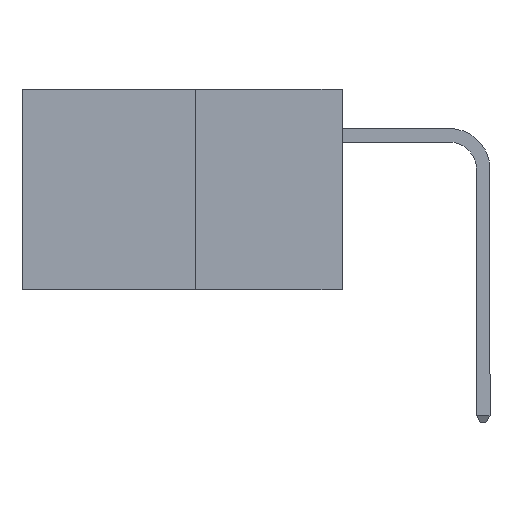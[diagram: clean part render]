
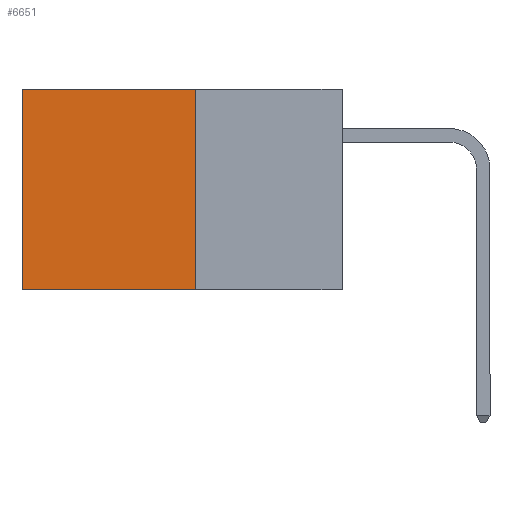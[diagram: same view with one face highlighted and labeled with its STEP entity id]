
A CAD part, left-side view. The second image highlights one B-rep face of the part: STEP entity #6651.
In plain terms, the highlighted planar face has unit normal (-1, 0, 0).
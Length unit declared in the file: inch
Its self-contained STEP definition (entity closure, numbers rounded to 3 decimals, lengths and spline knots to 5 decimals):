
#1680 = DIRECTION ( 'NONE',  ( 0., 0., -1. ) ) ;
#1918 = VERTEX_POINT ( 'NONE', #6724 ) ;
#2321 = VERTEX_POINT ( 'NONE', #21889 ) ;
#2814 = VERTEX_POINT ( 'NONE', #12919 ) ;
#4074 = DIRECTION ( 'NONE',  ( 0., 1., 0. ) ) ;
#5026 = EDGE_CURVE ( 'NONE', #2814, #1918, #20835, .T. ) ;
#5710 = ORIENTED_EDGE ( 'NONE', *, *, #10222, .F. ) ;
#6615 = LINE ( 'NONE', #10539, #15986 ) ;
#6651 = ADVANCED_FACE ( 'NONE', ( #14826 ), #9580, .F. ) ;
#6724 = CARTESIAN_POINT ( 'NONE',  ( 0.277, 0.59, 0. ) ) ;
#8294 = AXIS2_PLACEMENT_3D ( 'NONE', #15497, #8784, #8706 ) ;
#8706 = DIRECTION ( 'NONE',  ( 0., 0., -1. ) ) ;
#8784 = DIRECTION ( 'NONE',  ( 1., 0., 0. ) ) ;
#9580 = PLANE ( 'NONE',  #8294 ) ;
#9898 = CARTESIAN_POINT ( 'NONE',  ( 0.277, 0.27, 0. ) ) ;
#9905 = CARTESIAN_POINT ( 'NONE',  ( 0.277, 0.59, -0.37 ) ) ;
#10222 = EDGE_CURVE ( 'NONE', #2321, #20116, #14218, .T. ) ;
#10539 = CARTESIAN_POINT ( 'NONE',  ( 0.277, 0.27, -0.37 ) ) ;
#11614 = VECTOR ( 'NONE', #16657, 39.37008 ) ;
#11790 = EDGE_LOOP ( 'NONE', ( #13948, #5710, #15929, #20528 ) ) ;
#12919 = CARTESIAN_POINT ( 'NONE',  ( 0.277, 0.27, 0. ) ) ;
#13169 = CARTESIAN_POINT ( 'NONE',  ( 0.277, 0.59, -0.37 ) ) ;
#13433 = DIRECTION ( 'NONE',  ( 0., 0., -1. ) ) ;
#13948 = ORIENTED_EDGE ( 'NONE', *, *, #19528, .T. ) ;
#14218 = LINE ( 'NONE', #18161, #18277 ) ;
#14826 = FACE_OUTER_BOUND ( 'NONE', #11790, .T. ) ;
#15497 = CARTESIAN_POINT ( 'NONE',  ( 0.277, 0.27, -0.37 ) ) ;
#15929 = ORIENTED_EDGE ( 'NONE', *, *, #21591, .F. ) ;
#15986 = VECTOR ( 'NONE', #1680, 39.37008 ) ;
#16657 = DIRECTION ( 'NONE',  ( 0., 1., 0. ) ) ;
#17171 = VECTOR ( 'NONE', #13433, 39.37008 ) ;
#18161 = CARTESIAN_POINT ( 'NONE',  ( 0.277, 0.27, -0.37 ) ) ;
#18277 = VECTOR ( 'NONE', #4074, 39.37008 ) ;
#19528 = EDGE_CURVE ( 'NONE', #1918, #20116, #21713, .T. ) ;
#20116 = VERTEX_POINT ( 'NONE', #13169 ) ;
#20528 = ORIENTED_EDGE ( 'NONE', *, *, #5026, .T. ) ;
#20835 = LINE ( 'NONE', #9898, #11614 ) ;
#21591 = EDGE_CURVE ( 'NONE', #2814, #2321, #6615, .T. ) ;
#21713 = LINE ( 'NONE', #9905, #17171 ) ;
#21889 = CARTESIAN_POINT ( 'NONE',  ( 0.277, 0.27, -0.37 ) ) ;
